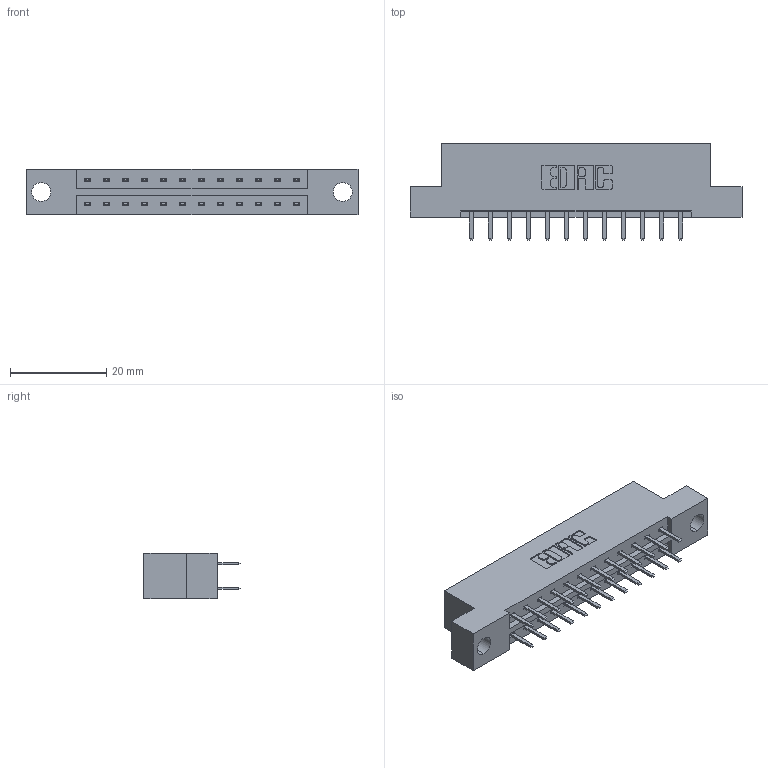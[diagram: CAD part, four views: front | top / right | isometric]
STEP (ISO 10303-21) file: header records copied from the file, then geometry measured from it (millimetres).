
FILE_DESCRIPTION (( 'STEP AP203' ), '1' );
FILE_NAME ('833-024-520-204.STEP', '2020-06-01T20:12:30', ( '' ), ( '' ), 'SwSTEP 2.0', 'SolidWorks 2020', '' );
FILE_SCHEMA (( 'CONFIG_CONTROL_DESIGN' ));
Length unit declared in the file: inch
Products named in the file (3): 833-024-520-204; 345-292-001_345-293-120; 833 Part_Flush - .156 Dia - TH
Assembly tree (25 placements, depth 2):
  833-024-520-204
    833 Part_Flush - .156 Dia - TH
    345-292-001_345-293-120  x24
Bounding box: 69.09 x 20.02 x 9.4 mm (x, y, z)
Volume: 6674.5 mm3; surface area: 7340.1 mm2
Topology: 25 solids, 25 shells, 1458 faces, 4223 edges, 2750 vertices
Faces by surface type: plane 982, cylinder 476
Entity records: 11717 total; most frequent: CARTESIAN_POINT 1990, ORIENTED_EDGE 1914, DIRECTION 1741, EDGE_CURVE 957, LINE 825, VECTOR 825, VERTEX_POINT 634, AXIS2_PLACEMENT_3D 458
